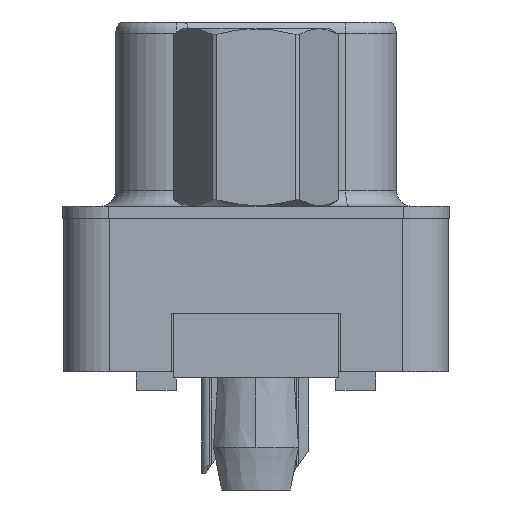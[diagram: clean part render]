
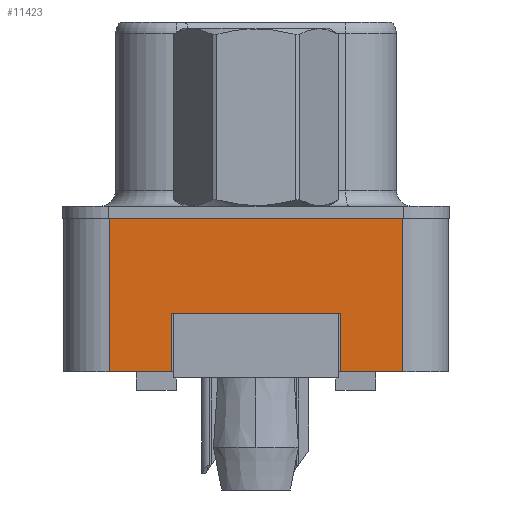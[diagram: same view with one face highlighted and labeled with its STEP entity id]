
A CAD part, left-side view. The second image highlights one B-rep face of the part: STEP entity #11423.
In plain terms, the highlighted planar face has unit normal (-1, 0, 0).
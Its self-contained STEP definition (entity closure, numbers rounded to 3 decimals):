
#1102 = VECTOR ( 'NONE', #7080, 1000. ) ;
#1165 = VECTOR ( 'NONE', #5310, 1000. ) ;
#1435 = CARTESIAN_POINT ( 'NONE',  ( -2.91, -4.775, -5. ) ) ;
#1953 = EDGE_CURVE ( 'NONE', #4052, #31547, #24770, .T. ) ;
#2735 = ORIENTED_EDGE ( 'NONE', *, *, #1953, .F. ) ;
#2990 = VERTEX_POINT ( 'NONE', #22799 ) ;
#3531 = ORIENTED_EDGE ( 'NONE', *, *, #32849, .T. ) ;
#3836 = VECTOR ( 'NONE', #22882, 1000. ) ;
#4052 = VERTEX_POINT ( 'NONE', #32875 ) ;
#4444 = EDGE_CURVE ( 'NONE', #2990, #10476, #11119, .T. ) ;
#4616 = ORIENTED_EDGE ( 'NONE', *, *, #19560, .T. ) ;
#5310 = DIRECTION ( 'NONE',  ( 0., 0., -1. ) ) ;
#5816 = ORIENTED_EDGE ( 'NONE', *, *, #22160, .T. ) ;
#6490 = DIRECTION ( 'NONE',  ( 0., -1., 0. ) ) ;
#6594 = VECTOR ( 'NONE', #16569, 1000. ) ;
#6902 = FACE_OUTER_BOUND ( 'NONE', #18703, .T. ) ;
#7080 = DIRECTION ( 'NONE',  ( 0., -1., 0. ) ) ;
#7930 = CARTESIAN_POINT ( 'NONE',  ( -2.91, -4.775, -5. ) ) ;
#9406 = VERTEX_POINT ( 'NONE', #15327 ) ;
#9492 = LINE ( 'NONE', #27670, #1102 ) ;
#9633 = DIRECTION ( 'NONE',  ( 0., 0., 1. ) ) ;
#9751 = VECTOR ( 'NONE', #6490, 1000. ) ;
#10476 = VERTEX_POINT ( 'NONE', #16723 ) ;
#10610 = CARTESIAN_POINT ( 'NONE',  ( -2.91, -2.75, -3.1 ) ) ;
#11119 = LINE ( 'NONE', #10610, #1165 ) ;
#11423 = ADVANCED_FACE ( 'NONE', ( #6902 ), #27331, .T. ) ;
#11866 = DIRECTION ( 'NONE',  ( -1., 0., 0. ) ) ;
#12026 = VECTOR ( 'NONE', #14401, 1000. ) ;
#14401 = DIRECTION ( 'NONE',  ( 0., 1., 0. ) ) ;
#14518 = CARTESIAN_POINT ( 'NONE',  ( -2.91, 2.75, -3.1 ) ) ;
#15327 = CARTESIAN_POINT ( 'NONE',  ( -2.91, -4.775, -5. ) ) ;
#16399 = VERTEX_POINT ( 'NONE', #32677 ) ;
#16569 = DIRECTION ( 'NONE',  ( 0., 0., -1. ) ) ;
#16612 = CARTESIAN_POINT ( 'NONE',  ( -2.91, 2.75, -3.1 ) ) ;
#16723 = CARTESIAN_POINT ( 'NONE',  ( -2.91, -2.75, -5. ) ) ;
#16748 = VECTOR ( 'NONE', #28000, 1000. ) ;
#17626 = CARTESIAN_POINT ( 'NONE',  ( -2.91, -4.775, 0. ) ) ;
#18703 = EDGE_LOOP ( 'NONE', ( #32476, #5816, #4616, #24793, #2735, #3531, #26150, #26482 ) ) ;
#19560 = EDGE_CURVE ( 'NONE', #9406, #16399, #20185, .T. ) ;
#19661 = CARTESIAN_POINT ( 'NONE',  ( -2.91, 2.75, -5. ) ) ;
#20185 = LINE ( 'NONE', #7930, #16748 ) ;
#21845 = VERTEX_POINT ( 'NONE', #28274 ) ;
#22034 = VECTOR ( 'NONE', #27977, 1000. ) ;
#22160 = EDGE_CURVE ( 'NONE', #10476, #9406, #24523, .T. ) ;
#22317 = LINE ( 'NONE', #14518, #6594 ) ;
#22799 = CARTESIAN_POINT ( 'NONE',  ( -2.91, -2.75, -3.1 ) ) ;
#22882 = DIRECTION ( 'NONE',  ( 0., -1., 0. ) ) ;
#24079 = EDGE_CURVE ( 'NONE', #21845, #30225, #22317, .T. ) ;
#24523 = LINE ( 'NONE', #29784, #9751 ) ;
#24770 = LINE ( 'NONE', #30195, #22034 ) ;
#24793 = ORIENTED_EDGE ( 'NONE', *, *, #32879, .F. ) ;
#24969 = AXIS2_PLACEMENT_3D ( 'NONE', #1435, #11866, #9633 ) ;
#25608 = LINE ( 'NONE', #17626, #3836 ) ;
#26150 = ORIENTED_EDGE ( 'NONE', *, *, #24079, .F. ) ;
#26482 = ORIENTED_EDGE ( 'NONE', *, *, #33117, .F. ) ;
#27331 = PLANE ( 'NONE',  #24969 ) ;
#27670 = CARTESIAN_POINT ( 'NONE',  ( -2.91, -4.775, -5. ) ) ;
#27977 = DIRECTION ( 'NONE',  ( 0., 0., 1. ) ) ;
#28000 = DIRECTION ( 'NONE',  ( 0., 0., 1. ) ) ;
#28274 = CARTESIAN_POINT ( 'NONE',  ( -2.91, 2.75, -3.1 ) ) ;
#29784 = CARTESIAN_POINT ( 'NONE',  ( -2.91, -4.775, -5. ) ) ;
#30116 = CARTESIAN_POINT ( 'NONE',  ( -2.91, 4.775, 0. ) ) ;
#30195 = CARTESIAN_POINT ( 'NONE',  ( -2.91, 4.775, -5. ) ) ;
#30225 = VERTEX_POINT ( 'NONE', #19661 ) ;
#31547 = VERTEX_POINT ( 'NONE', #30116 ) ;
#32410 = LINE ( 'NONE', #16612, #12026 ) ;
#32476 = ORIENTED_EDGE ( 'NONE', *, *, #4444, .T. ) ;
#32677 = CARTESIAN_POINT ( 'NONE',  ( -2.91, -4.775, 0. ) ) ;
#32849 = EDGE_CURVE ( 'NONE', #4052, #30225, #9492, .T. ) ;
#32875 = CARTESIAN_POINT ( 'NONE',  ( -2.91, 4.775, -5. ) ) ;
#32879 = EDGE_CURVE ( 'NONE', #31547, #16399, #25608, .T. ) ;
#33117 = EDGE_CURVE ( 'NONE', #2990, #21845, #32410, .T. ) ;
